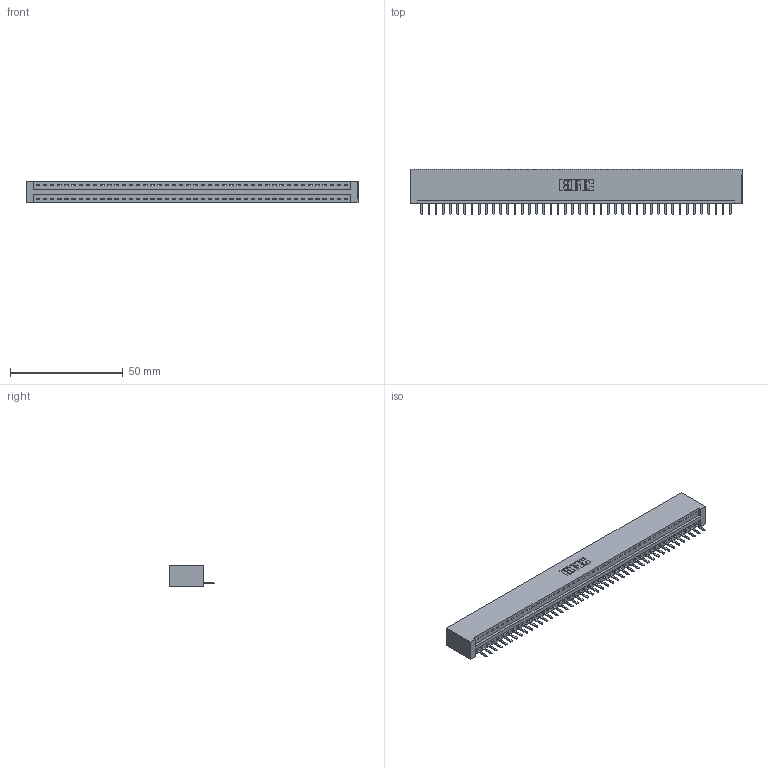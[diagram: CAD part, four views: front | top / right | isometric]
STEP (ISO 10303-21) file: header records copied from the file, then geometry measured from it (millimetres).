
FILE_DESCRIPTION (( 'STEP AP203' ), '1' );
FILE_NAME ('346-044-520-101.STEP', '2022-05-09T16:34:43', ( '' ), ( '' ), 'SwSTEP 2.0', 'SolidWorks 2020', '' );
FILE_SCHEMA (( 'CONFIG_CONTROL_DESIGN' ));
Length unit declared in the file: inch
Products named in the file (3): 346 Part_No Mounting Lugs; 345-292-001_345-293-120; 346-044-520-101
Assembly tree (45 placements, depth 2):
  346-044-520-101
    346 Part_No Mounting Lugs
    345-292-001_345-293-120  x44
Bounding box: 146.94 x 20.02 x 9.4 mm (x, y, z)
Volume: 14501.9 mm3; surface area: 17799.7 mm2
Topology: 45 solids, 45 shells, 2842 faces, 8401 edges, 5482 vertices
Faces by surface type: plane 1920, cylinder 922
Entity records: 26875 total; most frequent: CARTESIAN_POINT 4624, ORIENTED_EDGE 4590, DIRECTION 4059, EDGE_CURVE 2295, VECTOR 1991, LINE 1991, VERTEX_POINT 1526, AXIS2_PLACEMENT_3D 1034
